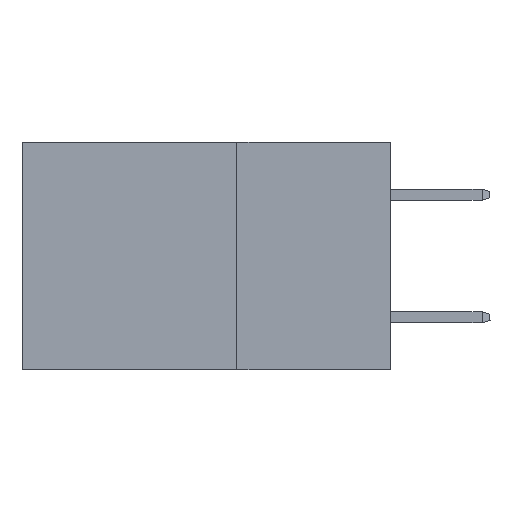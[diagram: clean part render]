
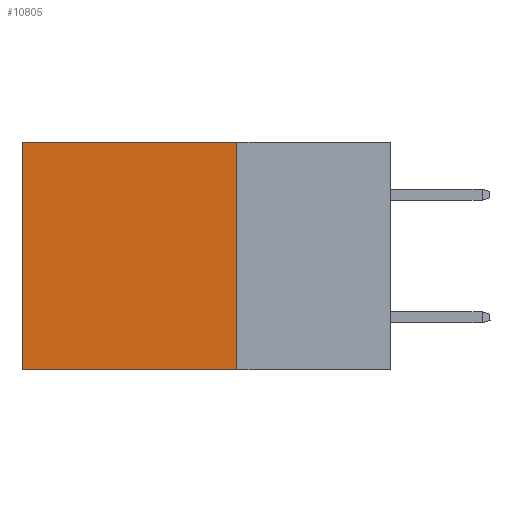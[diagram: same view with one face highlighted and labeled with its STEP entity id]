
A CAD part, left-side view. The second image highlights one B-rep face of the part: STEP entity #10805.
In plain terms, the highlighted planar face has unit normal (-1, 0, 0).
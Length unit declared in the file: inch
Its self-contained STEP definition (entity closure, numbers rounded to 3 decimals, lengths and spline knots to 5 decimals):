
#632 = EDGE_CURVE ( 'NONE', #4285, #26348, #4259, .T. ) ;
#812 = PLANE ( 'NONE',  #23177 ) ;
#1276 = DIRECTION ( 'NONE',  ( 0., 1., 0. ) ) ;
#1445 = ORIENTED_EDGE ( 'NONE', *, *, #632, .T. ) ;
#3441 = LINE ( 'NONE', #15964, #10485 ) ;
#4259 = LINE ( 'NONE', #19049, #7222 ) ;
#4285 = VERTEX_POINT ( 'NONE', #19908 ) ;
#4326 = CARTESIAN_POINT ( 'NONE',  ( 0.2875, 0.6, 0. ) ) ;
#4569 = EDGE_LOOP ( 'NONE', ( #25805, #15675, #10971, #1445 ) ) ;
#4665 = EDGE_CURVE ( 'NONE', #4285, #16500, #3441, .T. ) ;
#4684 = DIRECTION ( 'NONE',  ( 1., 0., 0. ) ) ;
#4858 = EDGE_CURVE ( 'NONE', #16500, #14590, #14244, .T. ) ;
#6990 = DIRECTION ( 'NONE',  ( 0., 0., -1. ) ) ;
#7222 = VECTOR ( 'NONE', #10410, 39.37008 ) ;
#7429 = DIRECTION ( 'NONE',  ( 0., 0., -1. ) ) ;
#8087 = VECTOR ( 'NONE', #1276, 39.37008 ) ;
#10410 = DIRECTION ( 'NONE',  ( 0., 1., 0. ) ) ;
#10485 = VECTOR ( 'NONE', #7429, 39.37008 ) ;
#10805 = ADVANCED_FACE ( 'NONE', ( #16147 ), #812, .F. ) ;
#10971 = ORIENTED_EDGE ( 'NONE', *, *, #4665, .F. ) ;
#14244 = LINE ( 'NONE', #21036, #8087 ) ;
#14348 = VECTOR ( 'NONE', #19967, 39.37008 ) ;
#14590 = VERTEX_POINT ( 'NONE', #20766 ) ;
#15675 = ORIENTED_EDGE ( 'NONE', *, *, #4858, .F. ) ;
#15964 = CARTESIAN_POINT ( 'NONE',  ( 0.2875, 0.25, 0. ) ) ;
#16147 = FACE_OUTER_BOUND ( 'NONE', #4569, .T. ) ;
#16500 = VERTEX_POINT ( 'NONE', #16902 ) ;
#16902 = CARTESIAN_POINT ( 'NONE',  ( 0.2875, 0.25, -0.37 ) ) ;
#18061 = LINE ( 'NONE', #24592, #14348 ) ;
#18450 = EDGE_CURVE ( 'NONE', #26348, #14590, #18061, .T. ) ;
#19049 = CARTESIAN_POINT ( 'NONE',  ( 0.2875, 0.25, 0. ) ) ;
#19908 = CARTESIAN_POINT ( 'NONE',  ( 0.2875, 0.25, 0. ) ) ;
#19967 = DIRECTION ( 'NONE',  ( 0., 0., -1. ) ) ;
#20766 = CARTESIAN_POINT ( 'NONE',  ( 0.2875, 0.6, -0.37 ) ) ;
#21036 = CARTESIAN_POINT ( 'NONE',  ( 0.2875, 0.25, -0.37 ) ) ;
#23177 = AXIS2_PLACEMENT_3D ( 'NONE', #24234, #4684, #6990 ) ;
#24234 = CARTESIAN_POINT ( 'NONE',  ( 0.2875, 0.25, 0. ) ) ;
#24592 = CARTESIAN_POINT ( 'NONE',  ( 0.2875, 0.6, 0. ) ) ;
#25805 = ORIENTED_EDGE ( 'NONE', *, *, #18450, .T. ) ;
#26348 = VERTEX_POINT ( 'NONE', #4326 ) ;
